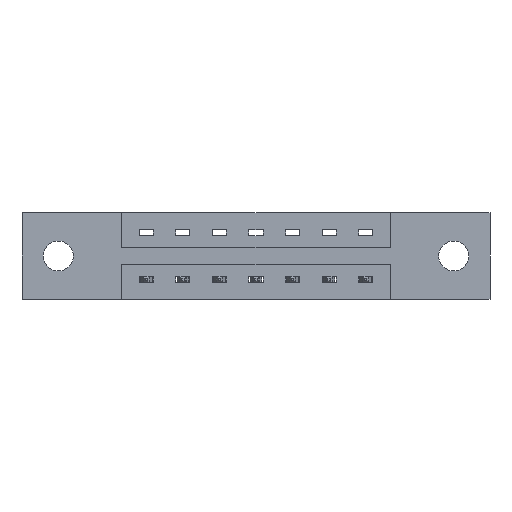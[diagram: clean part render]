
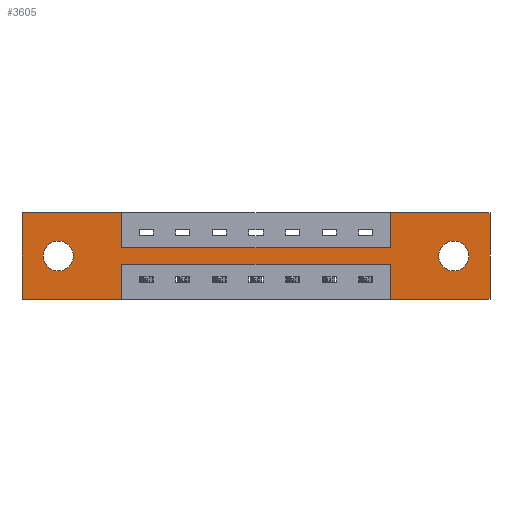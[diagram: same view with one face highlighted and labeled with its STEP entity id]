
A CAD part, front view. The second image highlights one B-rep face of the part: STEP entity #3605.
In plain terms, the highlighted planar face has unit normal (0, -1, 0).
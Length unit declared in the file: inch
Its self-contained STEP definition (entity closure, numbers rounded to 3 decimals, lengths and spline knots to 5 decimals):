
#128 = DIRECTION ( 'NONE',  ( 1., 0., 0. ) ) ;
#272 = VERTEX_POINT ( 'NONE', #2937 ) ;
#402 = CARTESIAN_POINT ( 'NONE',  ( 0., 0., 0. ) ) ;
#436 = ORIENTED_EDGE ( 'NONE', *, *, #4018, .F. ) ;
#582 = CIRCLE ( 'NONE', #8992, 0.064 ) ;
#599 = CARTESIAN_POINT ( 'NONE',  ( 1.843, 0., -0.121 ) ) ;
#682 = VECTOR ( 'NONE', #5595, 39.37008 ) ;
#782 = VERTEX_POINT ( 'NONE', #2792 ) ;
#844 = VERTEX_POINT ( 'NONE', #5340 ) ;
#907 = EDGE_CURVE ( 'NONE', #5432, #782, #9579, .T. ) ;
#964 = EDGE_CURVE ( 'NONE', #5140, #5053, #4642, .T. ) ;
#1200 = CARTESIAN_POINT ( 'NONE',  ( 0.425, 0., -0.22 ) ) ;
#1243 = ORIENTED_EDGE ( 'NONE', *, *, #4402, .F. ) ;
#1334 = EDGE_CURVE ( 'NONE', #6733, #5432, #6839, .T. ) ;
#1382 = CARTESIAN_POINT ( 'NONE',  ( 0.425, 0., -0.15 ) ) ;
#1385 = FACE_BOUND ( 'NONE', #2306, .T. ) ;
#1664 = CIRCLE ( 'NONE', #7179, 0.064 ) ;
#1702 = DIRECTION ( 'NONE',  ( 0., 1., 0. ) ) ;
#1712 = CARTESIAN_POINT ( 'NONE',  ( 0.155, 0., -0.185 ) ) ;
#1725 = CARTESIAN_POINT ( 'NONE',  ( 0.425, 0., -0.15 ) ) ;
#1796 = LINE ( 'NONE', #9313, #7788 ) ;
#1832 = DIRECTION ( 'NONE',  ( 1., 0., 0. ) ) ;
#2052 = VECTOR ( 'NONE', #7343, 39.37008 ) ;
#2058 = CARTESIAN_POINT ( 'NONE',  ( 0.425, 0., 0. ) ) ;
#2062 = EDGE_CURVE ( 'NONE', #6072, #5140, #4283, .T. ) ;
#2094 = PLANE ( 'NONE',  #3751 ) ;
#2098 = VECTOR ( 'NONE', #2201, 39.37008 ) ;
#2115 = VECTOR ( 'NONE', #2843, 39.37008 ) ;
#2134 = ORIENTED_EDGE ( 'NONE', *, *, #3025, .T. ) ;
#2183 = DIRECTION ( 'NONE',  ( 0., 0., -1. ) ) ;
#2197 = DIRECTION ( 'NONE',  ( 0., -1., 0. ) ) ;
#2201 = DIRECTION ( 'NONE',  ( 1., 0., 0. ) ) ;
#2260 = LINE ( 'NONE', #6123, #8243 ) ;
#2268 = LINE ( 'NONE', #1725, #9598 ) ;
#2306 = EDGE_LOOP ( 'NONE', ( #2369, #4394 ) ) ;
#2369 = ORIENTED_EDGE ( 'NONE', *, *, #4250, .T. ) ;
#2434 = EDGE_LOOP ( 'NONE', ( #2134, #6173 ) ) ;
#2458 = VECTOR ( 'NONE', #3909, 39.37008 ) ;
#2507 = VERTEX_POINT ( 'NONE', #2058 ) ;
#2595 = EDGE_CURVE ( 'NONE', #8780, #6733, #2268, .T. ) ;
#2792 = CARTESIAN_POINT ( 'NONE',  ( 1.998, 0., 0. ) ) ;
#2819 = ORIENTED_EDGE ( 'NONE', *, *, #3245, .F. ) ;
#2843 = DIRECTION ( 'NONE',  ( 0., 0., 1. ) ) ;
#2857 = VERTEX_POINT ( 'NONE', #5351 ) ;
#2887 = VECTOR ( 'NONE', #6304, 39.37008 ) ;
#2898 = LINE ( 'NONE', #3703, #2458 ) ;
#2937 = CARTESIAN_POINT ( 'NONE',  ( 0.155, 0., -0.121 ) ) ;
#3025 = EDGE_CURVE ( 'NONE', #4555, #844, #1664, .T. ) ;
#3042 = CARTESIAN_POINT ( 'NONE',  ( 0., 0., 0. ) ) ;
#3054 = ORIENTED_EDGE ( 'NONE', *, *, #907, .F. ) ;
#3197 = CARTESIAN_POINT ( 'NONE',  ( 1.573, 0., -0.37 ) ) ;
#3245 = EDGE_CURVE ( 'NONE', #8172, #6865, #2260, .T. ) ;
#3281 = ORIENTED_EDGE ( 'NONE', *, *, #7187, .F. ) ;
#3428 = CARTESIAN_POINT ( 'NONE',  ( 0., 0., -0.37 ) ) ;
#3471 = CARTESIAN_POINT ( 'NONE',  ( 0.155, 0., -0.249 ) ) ;
#3605 = ADVANCED_FACE ( 'NONE', ( #9275, #1385, #7204 ), #2094, .T. ) ;
#3686 = DIRECTION ( 'NONE',  ( 0., 0., 1. ) ) ;
#3703 = CARTESIAN_POINT ( 'NONE',  ( 1.998, 0., 0. ) ) ;
#3736 = DIRECTION ( 'NONE',  ( 0., 1., 0. ) ) ;
#3751 = AXIS2_PLACEMENT_3D ( 'NONE', #3428, #2197, #2183 ) ;
#3892 = DIRECTION ( 'NONE',  ( 0., 0., 1. ) ) ;
#3909 = DIRECTION ( 'NONE',  ( 0., 0., -1. ) ) ;
#4018 = EDGE_CURVE ( 'NONE', #2857, #6072, #1796, .T. ) ;
#4216 = DIRECTION ( 'NONE',  ( 0., 1., 0. ) ) ;
#4224 = CARTESIAN_POINT ( 'NONE',  ( 1.843, 0., -0.185 ) ) ;
#4250 = EDGE_CURVE ( 'NONE', #272, #8548, #582, .T. ) ;
#4283 = LINE ( 'NONE', #4799, #2052 ) ;
#4394 = ORIENTED_EDGE ( 'NONE', *, *, #5763, .T. ) ;
#4402 = EDGE_CURVE ( 'NONE', #2507, #8780, #7533, .T. ) ;
#4555 = VERTEX_POINT ( 'NONE', #599 ) ;
#4585 = CARTESIAN_POINT ( 'NONE',  ( 1.573, 0., 0. ) ) ;
#4642 = LINE ( 'NONE', #9137, #8332 ) ;
#4799 = CARTESIAN_POINT ( 'NONE',  ( 0.425, 0., -0.37 ) ) ;
#5014 = CARTESIAN_POINT ( 'NONE',  ( 1.573, 0., -0.37 ) ) ;
#5017 = DIRECTION ( 'NONE',  ( 0., 0., -1. ) ) ;
#5053 = VERTEX_POINT ( 'NONE', #5488 ) ;
#5065 = VERTEX_POINT ( 'NONE', #5993 ) ;
#5126 = ORIENTED_EDGE ( 'NONE', *, *, #1334, .F. ) ;
#5140 = VERTEX_POINT ( 'NONE', #5326 ) ;
#5326 = CARTESIAN_POINT ( 'NONE',  ( 0.425, 0., -0.37 ) ) ;
#5340 = CARTESIAN_POINT ( 'NONE',  ( 1.843, 0., -0.249 ) ) ;
#5351 = CARTESIAN_POINT ( 'NONE',  ( 1.573, 0., -0.22 ) ) ;
#5352 = EDGE_CURVE ( 'NONE', #844, #4555, #7191, .T. ) ;
#5378 = ORIENTED_EDGE ( 'NONE', *, *, #5866, .F. ) ;
#5432 = VERTEX_POINT ( 'NONE', #4585 ) ;
#5488 = CARTESIAN_POINT ( 'NONE',  ( 0., 0., -0.37 ) ) ;
#5569 = CARTESIAN_POINT ( 'NONE',  ( 1.573, 0., 0. ) ) ;
#5595 = DIRECTION ( 'NONE',  ( 0., 0., 1. ) ) ;
#5747 = AXIS2_PLACEMENT_3D ( 'NONE', #1712, #1702, #3892 ) ;
#5763 = EDGE_CURVE ( 'NONE', #8548, #272, #6842, .T. ) ;
#5866 = EDGE_CURVE ( 'NONE', #5053, #5065, #8099, .T. ) ;
#5993 = CARTESIAN_POINT ( 'NONE',  ( 0., 0., 0. ) ) ;
#6072 = VERTEX_POINT ( 'NONE', #1200 ) ;
#6082 = EDGE_CURVE ( 'NONE', #782, #8172, #2898, .T. ) ;
#6123 = CARTESIAN_POINT ( 'NONE',  ( 0., 0., -0.37 ) ) ;
#6173 = ORIENTED_EDGE ( 'NONE', *, *, #5352, .T. ) ;
#6304 = DIRECTION ( 'NONE',  ( 0., 0., 1. ) ) ;
#6403 = AXIS2_PLACEMENT_3D ( 'NONE', #4224, #4216, #5017 ) ;
#6516 = EDGE_CURVE ( 'NONE', #6865, #2857, #9028, .T. ) ;
#6646 = ORIENTED_EDGE ( 'NONE', *, *, #6516, .F. ) ;
#6733 = VERTEX_POINT ( 'NONE', #9284 ) ;
#6839 = LINE ( 'NONE', #5569, #682 ) ;
#6842 = CIRCLE ( 'NONE', #5747, 0.064 ) ;
#6864 = ORIENTED_EDGE ( 'NONE', *, *, #6082, .F. ) ;
#6865 = VERTEX_POINT ( 'NONE', #5014 ) ;
#7179 = AXIS2_PLACEMENT_3D ( 'NONE', #7843, #7682, #7717 ) ;
#7187 = EDGE_CURVE ( 'NONE', #5065, #2507, #8085, .T. ) ;
#7191 = CIRCLE ( 'NONE', #6403, 0.064 ) ;
#7204 = FACE_OUTER_BOUND ( 'NONE', #9113, .T. ) ;
#7343 = DIRECTION ( 'NONE',  ( 0., 0., -1. ) ) ;
#7527 = VECTOR ( 'NONE', #128, 39.37008 ) ;
#7533 = LINE ( 'NONE', #8655, #9379 ) ;
#7674 = CARTESIAN_POINT ( 'NONE',  ( 1.998, 0., -0.37 ) ) ;
#7682 = DIRECTION ( 'NONE',  ( 0., 1., 0. ) ) ;
#7717 = DIRECTION ( 'NONE',  ( 0., 0., -1. ) ) ;
#7788 = VECTOR ( 'NONE', #9659, 39.37008 ) ;
#7843 = CARTESIAN_POINT ( 'NONE',  ( 1.843, 0., -0.185 ) ) ;
#8085 = LINE ( 'NONE', #8834, #2098 ) ;
#8099 = LINE ( 'NONE', #402, #2115 ) ;
#8167 = CARTESIAN_POINT ( 'NONE',  ( 0.155, 0., -0.185 ) ) ;
#8172 = VERTEX_POINT ( 'NONE', #7674 ) ;
#8243 = VECTOR ( 'NONE', #9712, 39.37008 ) ;
#8309 = DIRECTION ( 'NONE',  ( -1., 0., 0. ) ) ;
#8332 = VECTOR ( 'NONE', #8309, 39.37008 ) ;
#8338 = ORIENTED_EDGE ( 'NONE', *, *, #2062, .F. ) ;
#8548 = VERTEX_POINT ( 'NONE', #3471 ) ;
#8652 = DIRECTION ( 'NONE',  ( 0., 0., -1. ) ) ;
#8655 = CARTESIAN_POINT ( 'NONE',  ( 0.425, 0., 0. ) ) ;
#8780 = VERTEX_POINT ( 'NONE', #1382 ) ;
#8834 = CARTESIAN_POINT ( 'NONE',  ( 0., 0., 0. ) ) ;
#8958 = ORIENTED_EDGE ( 'NONE', *, *, #2595, .F. ) ;
#8992 = AXIS2_PLACEMENT_3D ( 'NONE', #8167, #3736, #3686 ) ;
#9028 = LINE ( 'NONE', #3197, #2887 ) ;
#9113 = EDGE_LOOP ( 'NONE', ( #8338, #436, #6646, #2819, #6864, #3054, #5126, #8958, #1243, #3281, #5378, #9171 ) ) ;
#9137 = CARTESIAN_POINT ( 'NONE',  ( 0., 0., -0.37 ) ) ;
#9171 = ORIENTED_EDGE ( 'NONE', *, *, #964, .F. ) ;
#9275 = FACE_BOUND ( 'NONE', #2434, .T. ) ;
#9284 = CARTESIAN_POINT ( 'NONE',  ( 1.573, 0., -0.15 ) ) ;
#9313 = CARTESIAN_POINT ( 'NONE',  ( 0.425, 0., -0.22 ) ) ;
#9379 = VECTOR ( 'NONE', #8652, 39.37008 ) ;
#9579 = LINE ( 'NONE', #3042, #7527 ) ;
#9598 = VECTOR ( 'NONE', #1832, 39.37008 ) ;
#9659 = DIRECTION ( 'NONE',  ( -1., 0., 0. ) ) ;
#9712 = DIRECTION ( 'NONE',  ( -1., 0., 0. ) ) ;
